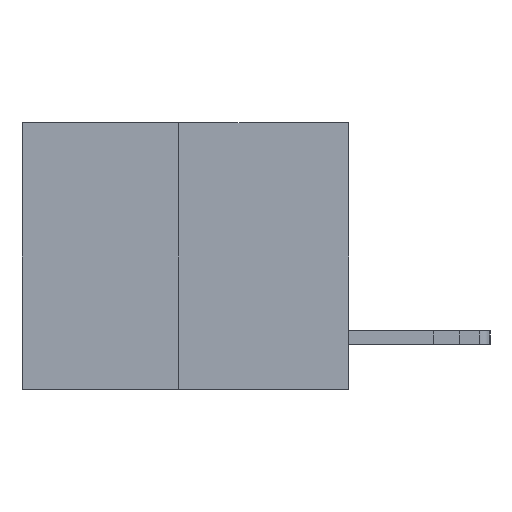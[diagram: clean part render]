
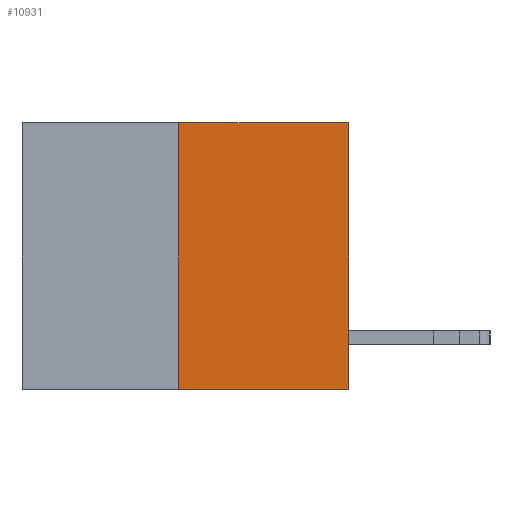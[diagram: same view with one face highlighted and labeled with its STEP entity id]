
A CAD part, left-side view. The second image highlights one B-rep face of the part: STEP entity #10931.
In plain terms, the highlighted planar face has unit normal (-1, 0, 0).
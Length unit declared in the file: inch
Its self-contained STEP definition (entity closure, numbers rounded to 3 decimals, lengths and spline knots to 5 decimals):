
#380 = VERTEX_POINT ( 'NONE', #6196 ) ;
#411 = VERTEX_POINT ( 'NONE', #6401 ) ;
#988 = DIRECTION ( 'NONE',  ( 0., -1., 0. ) ) ;
#2734 = CARTESIAN_POINT ( 'NONE',  ( 0., 0.6, -0.49 ) ) ;
#2868 = CARTESIAN_POINT ( 'NONE',  ( 0., 0., 0. ) ) ;
#3106 = AXIS2_PLACEMENT_3D ( 'NONE', #21286, #14881, #17655 ) ;
#3850 = LINE ( 'NONE', #5373, #16609 ) ;
#5373 = CARTESIAN_POINT ( 'NONE',  ( 0., 0.312, -0.49 ) ) ;
#6196 = CARTESIAN_POINT ( 'NONE',  ( 0., 0.312, 0. ) ) ;
#6401 = CARTESIAN_POINT ( 'NONE',  ( 0., 0., -0.49 ) ) ;
#8050 = DIRECTION ( 'NONE',  ( 0., 0., 1. ) ) ;
#8168 = VECTOR ( 'NONE', #11320, 39.37008 ) ;
#8900 = VECTOR ( 'NONE', #8050, 39.37008 ) ;
#9520 = ORIENTED_EDGE ( 'NONE', *, *, #10419, .F. ) ;
#9830 = ORIENTED_EDGE ( 'NONE', *, *, #11717, .T. ) ;
#9881 = ORIENTED_EDGE ( 'NONE', *, *, #20468, .F. ) ;
#10419 = EDGE_CURVE ( 'NONE', #380, #19695, #20114, .T. ) ;
#10756 = ORIENTED_EDGE ( 'NONE', *, *, #15884, .T. ) ;
#10931 = ADVANCED_FACE ( 'NONE', ( #18800 ), #11247, .F. ) ;
#11009 = LINE ( 'NONE', #2868, #8900 ) ;
#11247 = PLANE ( 'NONE',  #3106 ) ;
#11320 = DIRECTION ( 'NONE',  ( 0., -1., 0. ) ) ;
#11717 = EDGE_CURVE ( 'NONE', #16080, #411, #15359, .T. ) ;
#14307 = DIRECTION ( 'NONE',  ( 0., 0., 1. ) ) ;
#14881 = DIRECTION ( 'NONE',  ( 1., 0., 0. ) ) ;
#15359 = LINE ( 'NONE', #2734, #19813 ) ;
#15884 = EDGE_CURVE ( 'NONE', #411, #19695, #11009, .T. ) ;
#16080 = VERTEX_POINT ( 'NONE', #18019 ) ;
#16426 = CARTESIAN_POINT ( 'NONE',  ( 0., 0.6, 0. ) ) ;
#16609 = VECTOR ( 'NONE', #14307, 39.37008 ) ;
#17655 = DIRECTION ( 'NONE',  ( 0., 0., -1. ) ) ;
#18019 = CARTESIAN_POINT ( 'NONE',  ( 0., 0.312, -0.49 ) ) ;
#18800 = FACE_OUTER_BOUND ( 'NONE', #19516, .T. ) ;
#19516 = EDGE_LOOP ( 'NONE', ( #9881, #9830, #10756, #9520 ) ) ;
#19695 = VERTEX_POINT ( 'NONE', #20244 ) ;
#19813 = VECTOR ( 'NONE', #988, 39.37008 ) ;
#20114 = LINE ( 'NONE', #16426, #8168 ) ;
#20244 = CARTESIAN_POINT ( 'NONE',  ( 0., 0., 0. ) ) ;
#20468 = EDGE_CURVE ( 'NONE', #16080, #380, #3850, .T. ) ;
#21286 = CARTESIAN_POINT ( 'NONE',  ( 0., 0.6, 0. ) ) ;
